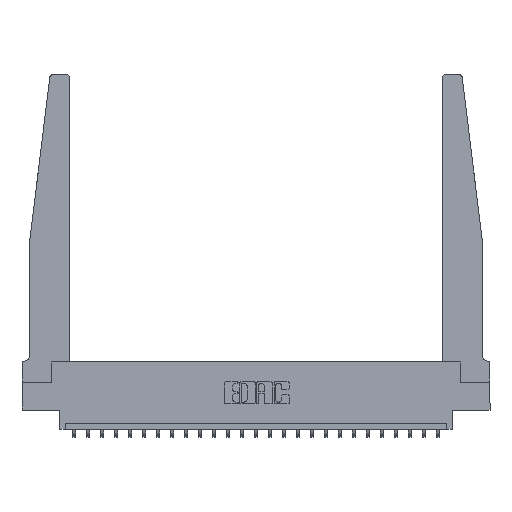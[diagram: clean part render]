
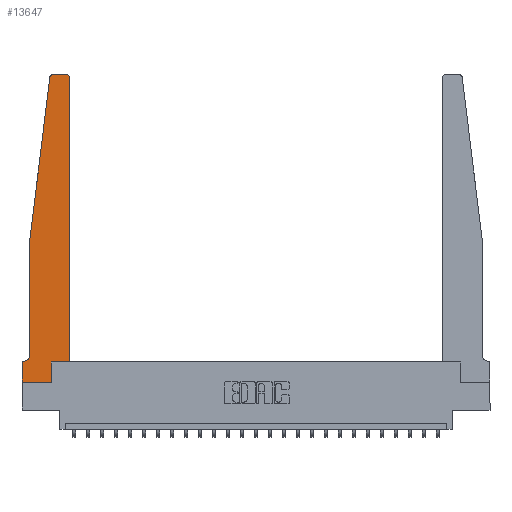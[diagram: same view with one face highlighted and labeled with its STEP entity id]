
A CAD part, top view. The second image highlights one B-rep face of the part: STEP entity #13647.
In plain terms, the highlighted planar face has unit normal (0, 0, 1).
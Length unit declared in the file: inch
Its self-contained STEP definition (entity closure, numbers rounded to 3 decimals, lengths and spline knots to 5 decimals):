
#36 = VERTEX_POINT ( 'NONE', #12276 ) ;
#194 = EDGE_CURVE ( 'NONE', #3594, #20026, #12886, .T. ) ;
#337 = EDGE_CURVE ( 'NONE', #16282, #21188, #19007, .T. ) ;
#491 = CARTESIAN_POINT ( 'NONE',  ( 0.27653, 2.72, 0.37 ) ) ;
#592 = DIRECTION ( 'NONE',  ( 0., 0., 1. ) ) ;
#790 = CARTESIAN_POINT ( 'NONE',  ( 0.425, 2.72, 0.37 ) ) ;
#1293 = FACE_OUTER_BOUND ( 'NONE', #8588, .T. ) ;
#1390 = VECTOR ( 'NONE', #5767, 39.37008 ) ;
#1515 = VECTOR ( 'NONE', #19002, 39.37008 ) ;
#2225 = EDGE_CURVE ( 'NONE', #10728, #12296, #2291, .T. ) ;
#2291 = LINE ( 'NONE', #13655, #17264 ) ;
#2334 = EDGE_CURVE ( 'NONE', #12296, #7046, #14920, .T. ) ;
#2467 = EDGE_CURVE ( 'NONE', #21188, #8798, #19711, .T. ) ;
#2756 = CIRCLE ( 'NONE', #12953, 0.03 ) ;
#3235 = LINE ( 'NONE', #22100, #23555 ) ;
#3594 = VERTEX_POINT ( 'NONE', #8152 ) ;
#4023 = EDGE_CURVE ( 'NONE', #7046, #18148, #17148, .T. ) ;
#4141 = DIRECTION ( 'NONE',  ( 0., 1., 0. ) ) ;
#4877 = VECTOR ( 'NONE', #21683, 39.37008 ) ;
#5033 = LINE ( 'NONE', #16766, #1390 ) ;
#5203 = PLANE ( 'NONE',  #11223 ) ;
#5332 = CARTESIAN_POINT ( 'NONE',  ( 0., 0.1875, 0.37 ) ) ;
#5397 = DIRECTION ( 'NONE',  ( -0.122, -0.992, 0. ) ) ;
#5411 = CARTESIAN_POINT ( 'NONE',  ( 0., 0., 0.37 ) ) ;
#5436 = DIRECTION ( 'NONE',  ( 0., 1., 0. ) ) ;
#5767 = DIRECTION ( 'NONE',  ( 1., 0., 0. ) ) ;
#6076 = ORIENTED_EDGE ( 'NONE', *, *, #2225, .T. ) ;
#6181 = CARTESIAN_POINT ( 'NONE',  ( 0.395, 2.75, 0.37 ) ) ;
#6888 = CARTESIAN_POINT ( 'NONE',  ( 0., 0., 0.37 ) ) ;
#7046 = VERTEX_POINT ( 'NONE', #6181 ) ;
#7339 = EDGE_CURVE ( 'NONE', #18148, #14438, #2756, .T. ) ;
#7698 = VECTOR ( 'NONE', #8498, 39.37008 ) ;
#7778 = CARTESIAN_POINT ( 'NONE',  ( 0.065, 1.25, 0.37 ) ) ;
#7889 = ORIENTED_EDGE ( 'NONE', *, *, #194, .T. ) ;
#8152 = CARTESIAN_POINT ( 'NONE',  ( 0.2605, 0., 0.37 ) ) ;
#8498 = DIRECTION ( 'NONE',  ( 0., -1., 0. ) ) ;
#8588 = EDGE_LOOP ( 'NONE', ( #13173, #12560, #17556, #12157, #16389, #11185, #9834, #15084, #7889, #15005, #6076, #10035 ) ) ;
#8615 = LINE ( 'NONE', #11891, #7698 ) ;
#8798 = VERTEX_POINT ( 'NONE', #24017 ) ;
#8920 = VECTOR ( 'NONE', #5397, 39.37008 ) ;
#8924 = EDGE_CURVE ( 'NONE', #10132, #3594, #16036, .T. ) ;
#8934 = EDGE_CURVE ( 'NONE', #20026, #10728, #5033, .T. ) ;
#9162 = AXIS2_PLACEMENT_3D ( 'NONE', #14627, #22126, #16226 ) ;
#9834 = ORIENTED_EDGE ( 'NONE', *, *, #9897, .T. ) ;
#9897 = EDGE_CURVE ( 'NONE', #36, #10132, #8615, .T. ) ;
#10035 = ORIENTED_EDGE ( 'NONE', *, *, #2334, .T. ) ;
#10132 = VERTEX_POINT ( 'NONE', #5411 ) ;
#10236 = CARTESIAN_POINT ( 'NONE',  ( 0.425, 0.18, 0.37 ) ) ;
#10708 = DIRECTION ( 'NONE',  ( 0., 0., 1. ) ) ;
#10728 = VERTEX_POINT ( 'NONE', #10236 ) ;
#11185 = ORIENTED_EDGE ( 'NONE', *, *, #21508, .T. ) ;
#11223 = AXIS2_PLACEMENT_3D ( 'NONE', #5332, #10708, #23811 ) ;
#11891 = CARTESIAN_POINT ( 'NONE',  ( 0., 0., 0.37 ) ) ;
#12157 = ORIENTED_EDGE ( 'NONE', *, *, #337, .T. ) ;
#12276 = CARTESIAN_POINT ( 'NONE',  ( 0., 0.1875, 0.37 ) ) ;
#12296 = VERTEX_POINT ( 'NONE', #790 ) ;
#12317 = VECTOR ( 'NONE', #21210, 39.37008 ) ;
#12560 = ORIENTED_EDGE ( 'NONE', *, *, #7339, .T. ) ;
#12886 = LINE ( 'NONE', #14717, #20854 ) ;
#12953 = AXIS2_PLACEMENT_3D ( 'NONE', #491, #15387, #19085 ) ;
#13104 = CARTESIAN_POINT ( 'NONE',  ( 0.27653, 2.75, 0.37 ) ) ;
#13173 = ORIENTED_EDGE ( 'NONE', *, *, #4023, .T. ) ;
#13647 = ADVANCED_FACE ( 'NONE', ( #1293 ), #5203, .T. ) ;
#13655 = CARTESIAN_POINT ( 'NONE',  ( 0.425, 0.18, 0.37 ) ) ;
#14114 = EDGE_CURVE ( 'NONE', #14438, #16282, #14671, .T. ) ;
#14438 = VERTEX_POINT ( 'NONE', #22834 ) ;
#14627 = CARTESIAN_POINT ( 'NONE',  ( 0.015, 0.2375, 0.37 ) ) ;
#14671 = LINE ( 'NONE', #16752, #8920 ) ;
#14717 = CARTESIAN_POINT ( 'NONE',  ( 0.2605, 0.18, 0.37 ) ) ;
#14920 = CIRCLE ( 'NONE', #16492, 0.03 ) ;
#15005 = ORIENTED_EDGE ( 'NONE', *, *, #8934, .T. ) ;
#15084 = ORIENTED_EDGE ( 'NONE', *, *, #8924, .T. ) ;
#15387 = DIRECTION ( 'NONE',  ( 0., 0., 1. ) ) ;
#15420 = CARTESIAN_POINT ( 'NONE',  ( 0.25, 2.75, 0.37 ) ) ;
#16036 = LINE ( 'NONE', #6888, #4877 ) ;
#16226 = DIRECTION ( 'NONE',  ( -1., 0., 0. ) ) ;
#16282 = VERTEX_POINT ( 'NONE', #17794 ) ;
#16389 = ORIENTED_EDGE ( 'NONE', *, *, #2467, .T. ) ;
#16492 = AXIS2_PLACEMENT_3D ( 'NONE', #17334, #592, #17098 ) ;
#16752 = CARTESIAN_POINT ( 'NONE',  ( 0.065, 1.25, 0.37 ) ) ;
#16766 = CARTESIAN_POINT ( 'NONE',  ( 0.425, 0.18, 0.37 ) ) ;
#17098 = DIRECTION ( 'NONE',  ( 1., 0., 0. ) ) ;
#17148 = LINE ( 'NONE', #15420, #1515 ) ;
#17264 = VECTOR ( 'NONE', #4141, 39.37008 ) ;
#17334 = CARTESIAN_POINT ( 'NONE',  ( 0.395, 2.72, 0.37 ) ) ;
#17556 = ORIENTED_EDGE ( 'NONE', *, *, #14114, .T. ) ;
#17794 = CARTESIAN_POINT ( 'NONE',  ( 0.065, 1.25, 0.37 ) ) ;
#18148 = VERTEX_POINT ( 'NONE', #13104 ) ;
#19002 = DIRECTION ( 'NONE',  ( -1., 0., 0. ) ) ;
#19007 = LINE ( 'NONE', #7778, #12317 ) ;
#19085 = DIRECTION ( 'NONE',  ( 1., 0., 0. ) ) ;
#19711 = CIRCLE ( 'NONE', #9162, 0.05 ) ;
#20026 = VERTEX_POINT ( 'NONE', #22127 ) ;
#20854 = VECTOR ( 'NONE', #5436, 39.37008 ) ;
#21188 = VERTEX_POINT ( 'NONE', #22006 ) ;
#21210 = DIRECTION ( 'NONE',  ( 0., -1., 0. ) ) ;
#21508 = EDGE_CURVE ( 'NONE', #8798, #36, #3235, .T. ) ;
#21683 = DIRECTION ( 'NONE',  ( 1., 0., 0. ) ) ;
#21850 = DIRECTION ( 'NONE',  ( -1., 0., 0. ) ) ;
#22006 = CARTESIAN_POINT ( 'NONE',  ( 0.065, 0.2375, 0.37 ) ) ;
#22100 = CARTESIAN_POINT ( 'NONE',  ( 0.065, 0.1875, 0.37 ) ) ;
#22126 = DIRECTION ( 'NONE',  ( 0., 0., -1. ) ) ;
#22127 = CARTESIAN_POINT ( 'NONE',  ( 0.2605, 0.18, 0.37 ) ) ;
#22834 = CARTESIAN_POINT ( 'NONE',  ( 0.24675, 2.72367, 0.37 ) ) ;
#23555 = VECTOR ( 'NONE', #21850, 39.37008 ) ;
#23811 = DIRECTION ( 'NONE',  ( 1., 0., 0. ) ) ;
#24017 = CARTESIAN_POINT ( 'NONE',  ( 0.015, 0.1875, 0.37 ) ) ;
